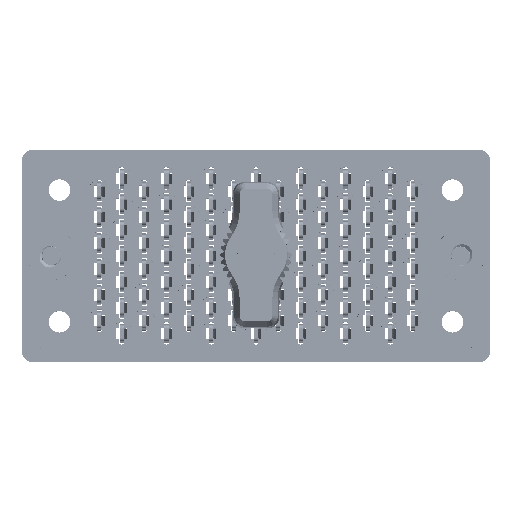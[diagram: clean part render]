
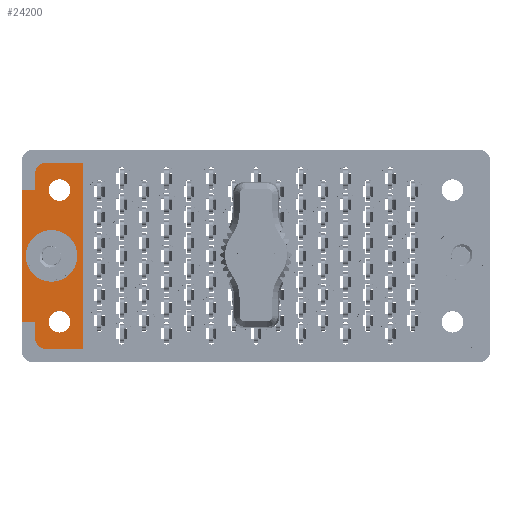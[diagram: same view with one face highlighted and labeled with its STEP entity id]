
A CAD part, top view. The second image highlights one B-rep face of the part: STEP entity #24200.
In plain terms, the highlighted planar face has unit normal (0, 0, 1).
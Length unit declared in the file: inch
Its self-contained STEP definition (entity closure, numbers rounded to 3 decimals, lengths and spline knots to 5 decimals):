
#584 = EDGE_CURVE ( 'NONE', #89817, #91354, #17436, .T. ) ;
#2251 = ORIENTED_EDGE ( 'NONE', *, *, #36343, .T. ) ;
#2655 = LINE ( 'NONE', #11920, #31902 ) ;
#2772 = DIRECTION ( 'NONE',  ( 1., 0., 0. ) ) ;
#2931 = CARTESIAN_POINT ( 'NONE',  ( -1.141, -0.3825, -0.117 ) ) ;
#3089 = CARTESIAN_POINT ( 'NONE',  ( -1.359, -0.617, -0.117 ) ) ;
#3422 = DIRECTION ( 'NONE',  ( 1., 0., 0. ) ) ;
#4078 = DIRECTION ( 'NONE',  ( -1., 0., 0. ) ) ;
#4494 = EDGE_LOOP ( 'NONE', ( #61712, #11989, #77170, #13019, #67879, #41958, #38583, #2251, #88502, #84819 ) ) ;
#4576 = VECTOR ( 'NONE', #77786, 39.37008 ) ;
#5213 = CARTESIAN_POINT ( 'NONE',  ( -1.2205, 0.54, -0.117 ) ) ;
#6321 = CARTESIAN_POINT ( 'NONE',  ( -1.005, -0.54, -0.117 ) ) ;
#6456 = DIRECTION ( 'NONE',  ( 0., -1., 0. ) ) ;
#7248 = DIRECTION ( 'NONE',  ( 0., 0., 1. ) ) ;
#7659 = VERTEX_POINT ( 'NONE', #25969 ) ;
#7745 = EDGE_CURVE ( 'NONE', #91354, #80050, #22111, .T. ) ;
#8574 = CARTESIAN_POINT ( 'NONE',  ( 0., -0.3825, -0.117 ) ) ;
#9942 = DIRECTION ( 'NONE',  ( 0., 0., 1. ) ) ;
#10424 = ORIENTED_EDGE ( 'NONE', *, *, #82706, .F. ) ;
#10697 = CARTESIAN_POINT ( 'NONE',  ( -1.005, 0.617, -0.117 ) ) ;
#11920 = CARTESIAN_POINT ( 'NONE',  ( -1.359, 0.617, -0.117 ) ) ;
#11989 = ORIENTED_EDGE ( 'NONE', *, *, #26077, .T. ) ;
#13019 = ORIENTED_EDGE ( 'NONE', *, *, #584, .T. ) ;
#13942 = EDGE_CURVE ( 'NONE', #76159, #19146, #96449, .T. ) ;
#14203 = CIRCLE ( 'NONE', #43000, 0.0625 ) ;
#14235 = FACE_OUTER_BOUND ( 'NONE', #4494, .T. ) ;
#14667 = LINE ( 'NONE', #84704, #37992 ) ;
#15086 = LINE ( 'NONE', #65351, #41941 ) ;
#17436 = LINE ( 'NONE', #10697, #4576 ) ;
#17962 = DIRECTION ( 'NONE',  ( 0., 0., 1. ) ) ;
#18045 = ORIENTED_EDGE ( 'NONE', *, *, #22325, .F. ) ;
#18982 = CARTESIAN_POINT ( 'NONE',  ( -1.359, -0.3825, -0.117 ) ) ;
#19146 = VERTEX_POINT ( 'NONE', #18982 ) ;
#21263 = DIRECTION ( 'NONE',  ( 0., 0., 1. ) ) ;
#21271 = FACE_BOUND ( 'NONE', #89228, .T. ) ;
#21396 = AXIS2_PLACEMENT_3D ( 'NONE', #3089, #9942, #2772 ) ;
#22111 = LINE ( 'NONE', #93864, #83931 ) ;
#22325 = EDGE_CURVE ( 'NONE', #70479, #45885, #48281, .T. ) ;
#22971 = CARTESIAN_POINT ( 'NONE',  ( 0., 0.3825, -0.117 ) ) ;
#23127 = ORIENTED_EDGE ( 'NONE', *, *, #91706, .F. ) ;
#23560 = DIRECTION ( 'NONE',  ( -1., 0., 0. ) ) ;
#24200 = ADVANCED_FACE ( 'NONE', ( #94797, #32881, #21271, #14235 ), #91572, .T. ) ;
#24434 = DIRECTION ( 'NONE',  ( 1., 0., 0. ) ) ;
#25859 = DIRECTION ( 'NONE',  ( 1., 0., 0. ) ) ;
#25969 = CARTESIAN_POINT ( 'NONE',  ( -1.359, 0.3825, -0.117 ) ) ;
#26077 = EDGE_CURVE ( 'NONE', #76765, #69805, #69997, .T. ) ;
#27530 = AXIS2_PLACEMENT_3D ( 'NONE', #59504, #43585, #81041 ) ;
#28534 = DIRECTION ( 'NONE',  ( 0., 0., 1. ) ) ;
#28970 = AXIS2_PLACEMENT_3D ( 'NONE', #69075, #53409, #24434 ) ;
#29681 = EDGE_CURVE ( 'NONE', #39636, #71266, #33413, .T. ) ;
#30223 = EDGE_CURVE ( 'NONE', #66978, #75219, #14667, .T. ) ;
#31685 = AXIS2_PLACEMENT_3D ( 'NONE', #49364, #78367, #3422 ) ;
#31902 = VECTOR ( 'NONE', #34444, 39.37008 ) ;
#32881 = FACE_BOUND ( 'NONE', #71653, .T. ) ;
#33216 = CARTESIAN_POINT ( 'NONE',  ( -1.2205, -0.54, -0.117 ) ) ;
#33413 = CIRCLE ( 'NONE', #31685, 0.15 ) ;
#34444 = DIRECTION ( 'NONE',  ( 0., -1., 0. ) ) ;
#34535 = DIRECTION ( 'NONE',  ( 0., -1., 0. ) ) ;
#36343 = EDGE_CURVE ( 'NONE', #75219, #7659, #60620, .T. ) ;
#36638 = DIRECTION ( 'NONE',  ( 1., 0., 0. ) ) ;
#37349 = EDGE_CURVE ( 'NONE', #76159, #76765, #80254, .T. ) ;
#37992 = VECTOR ( 'NONE', #34535, 39.37008 ) ;
#38459 = AXIS2_PLACEMENT_3D ( 'NONE', #95412, #28534, #36638 ) ;
#38583 = ORIENTED_EDGE ( 'NONE', *, *, #30223, .T. ) ;
#39359 = CARTESIAN_POINT ( 'NONE',  ( -1.0785, -0.3825, -0.117 ) ) ;
#39636 = VERTEX_POINT ( 'NONE', #50118 ) ;
#39891 = CARTESIAN_POINT ( 'NONE',  ( -1.141, 0.3825, -0.117 ) ) ;
#41569 = VERTEX_POINT ( 'NONE', #39359 ) ;
#41941 = VECTOR ( 'NONE', #88215, 39.37008 ) ;
#41958 = ORIENTED_EDGE ( 'NONE', *, *, #55975, .T. ) ;
#43000 = AXIS2_PLACEMENT_3D ( 'NONE', #2931, #17962, #70067 ) ;
#43077 = AXIS2_PLACEMENT_3D ( 'NONE', #58995, #21263, #59316 ) ;
#43585 = DIRECTION ( 'NONE',  ( 0., 0., 1. ) ) ;
#44831 = CIRCLE ( 'NONE', #88468, 0.0625 ) ;
#45885 = VERTEX_POINT ( 'NONE', #50500 ) ;
#47069 = CARTESIAN_POINT ( 'NONE',  ( -1.005, 0.54, -0.117 ) ) ;
#48281 = CIRCLE ( 'NONE', #43077, 0.0625 ) ;
#49057 = VERTEX_POINT ( 'NONE', #83991 ) ;
#49364 = CARTESIAN_POINT ( 'NONE',  ( -1.1875, 0., -0.117 ) ) ;
#49655 = VECTOR ( 'NONE', #23560, 39.37008 ) ;
#50118 = CARTESIAN_POINT ( 'NONE',  ( -1.3375, 0., -0.117 ) ) ;
#50500 = CARTESIAN_POINT ( 'NONE',  ( -1.0785, 0.3825, -0.117 ) ) ;
#51897 = CARTESIAN_POINT ( 'NONE',  ( -1.2205, 0.478, -0.117 ) ) ;
#51917 = ORIENTED_EDGE ( 'NONE', *, *, #59983, .F. ) ;
#51992 = CIRCLE ( 'NONE', #52500, 0.062 ) ;
#52500 = AXIS2_PLACEMENT_3D ( 'NONE', #51897, #7248, #59399 ) ;
#52892 = CIRCLE ( 'NONE', #27530, 0.15 ) ;
#53409 = DIRECTION ( 'NONE',  ( 0., 0., 1. ) ) ;
#53585 = VECTOR ( 'NONE', #90529, 39.37008 ) ;
#53590 = EDGE_LOOP ( 'NONE', ( #51917, #23127 ) ) ;
#54897 = ORIENTED_EDGE ( 'NONE', *, *, #88645, .F. ) ;
#55975 = EDGE_CURVE ( 'NONE', #80050, #66978, #51992, .T. ) ;
#56839 = CARTESIAN_POINT ( 'NONE',  ( -1.2825, 0.3825, -0.117 ) ) ;
#58995 = CARTESIAN_POINT ( 'NONE',  ( -1.141, 0.3825, -0.117 ) ) ;
#59316 = DIRECTION ( 'NONE',  ( 1., 0., 0. ) ) ;
#59399 = DIRECTION ( 'NONE',  ( 1., 0., 0. ) ) ;
#59504 = CARTESIAN_POINT ( 'NONE',  ( -1.1875, 0., -0.117 ) ) ;
#59983 = EDGE_CURVE ( 'NONE', #49057, #41569, #88556, .T. ) ;
#60620 = LINE ( 'NONE', #22971, #53585 ) ;
#61712 = ORIENTED_EDGE ( 'NONE', *, *, #37349, .T. ) ;
#63562 = CARTESIAN_POINT ( 'NONE',  ( -1.2825, 0., -0.117 ) ) ;
#65351 = CARTESIAN_POINT ( 'NONE',  ( 0., -0.54, -0.117 ) ) ;
#66978 = VERTEX_POINT ( 'NONE', #88793 ) ;
#67879 = ORIENTED_EDGE ( 'NONE', *, *, #7745, .T. ) ;
#68303 = CARTESIAN_POINT ( 'NONE',  ( -1.2825, -0.478, -0.117 ) ) ;
#69075 = CARTESIAN_POINT ( 'NONE',  ( -1.2205, -0.478, -0.117 ) ) ;
#69805 = VERTEX_POINT ( 'NONE', #33216 ) ;
#69997 = CIRCLE ( 'NONE', #28970, 0.062 ) ;
#70067 = DIRECTION ( 'NONE',  ( 1., 0., 0. ) ) ;
#70479 = VERTEX_POINT ( 'NONE', #86197 ) ;
#70659 = CARTESIAN_POINT ( 'NONE',  ( -1.2825, -0.3825, -0.117 ) ) ;
#71266 = VERTEX_POINT ( 'NONE', #85752 ) ;
#71653 = EDGE_LOOP ( 'NONE', ( #18045, #54897 ) ) ;
#75219 = VERTEX_POINT ( 'NONE', #56839 ) ;
#76159 = VERTEX_POINT ( 'NONE', #70659 ) ;
#76765 = VERTEX_POINT ( 'NONE', #68303 ) ;
#76794 = VECTOR ( 'NONE', #6456, 39.37008 ) ;
#77170 = ORIENTED_EDGE ( 'NONE', *, *, #86750, .F. ) ;
#77786 = DIRECTION ( 'NONE',  ( 0., 1., 0. ) ) ;
#78367 = DIRECTION ( 'NONE',  ( 0., 0., 1. ) ) ;
#80050 = VERTEX_POINT ( 'NONE', #5213 ) ;
#80254 = LINE ( 'NONE', #63562, #76794 ) ;
#81041 = DIRECTION ( 'NONE',  ( 1., 0., 0. ) ) ;
#82706 = EDGE_CURVE ( 'NONE', #71266, #39636, #52892, .T. ) ;
#83931 = VECTOR ( 'NONE', #4078, 39.37008 ) ;
#83991 = CARTESIAN_POINT ( 'NONE',  ( -1.2035, -0.3825, -0.117 ) ) ;
#84704 = CARTESIAN_POINT ( 'NONE',  ( -1.2825, 0., -0.117 ) ) ;
#84819 = ORIENTED_EDGE ( 'NONE', *, *, #13942, .F. ) ;
#85752 = CARTESIAN_POINT ( 'NONE',  ( -1.0375, 0., -0.117 ) ) ;
#86197 = CARTESIAN_POINT ( 'NONE',  ( -1.2035, 0.3825, -0.117 ) ) ;
#86750 = EDGE_CURVE ( 'NONE', #89817, #69805, #15086, .T. ) ;
#88215 = DIRECTION ( 'NONE',  ( -1., 0., 0. ) ) ;
#88468 = AXIS2_PLACEMENT_3D ( 'NONE', #39891, #92149, #25859 ) ;
#88502 = ORIENTED_EDGE ( 'NONE', *, *, #89691, .T. ) ;
#88556 = CIRCLE ( 'NONE', #38459, 0.0625 ) ;
#88645 = EDGE_CURVE ( 'NONE', #45885, #70479, #44831, .T. ) ;
#88793 = CARTESIAN_POINT ( 'NONE',  ( -1.2825, 0.478, -0.117 ) ) ;
#89228 = EDGE_LOOP ( 'NONE', ( #10424, #95014 ) ) ;
#89691 = EDGE_CURVE ( 'NONE', #7659, #19146, #2655, .T. ) ;
#89817 = VERTEX_POINT ( 'NONE', #6321 ) ;
#90529 = DIRECTION ( 'NONE',  ( -1., 0., 0. ) ) ;
#91354 = VERTEX_POINT ( 'NONE', #47069 ) ;
#91572 = PLANE ( 'NONE',  #21396 ) ;
#91706 = EDGE_CURVE ( 'NONE', #41569, #49057, #14203, .T. ) ;
#92149 = DIRECTION ( 'NONE',  ( 0., 0., 1. ) ) ;
#93864 = CARTESIAN_POINT ( 'NONE',  ( 0., 0.54, -0.117 ) ) ;
#94797 = FACE_BOUND ( 'NONE', #53590, .T. ) ;
#95014 = ORIENTED_EDGE ( 'NONE', *, *, #29681, .F. ) ;
#95412 = CARTESIAN_POINT ( 'NONE',  ( -1.141, -0.3825, -0.117 ) ) ;
#96449 = LINE ( 'NONE', #8574, #49655 ) ;
